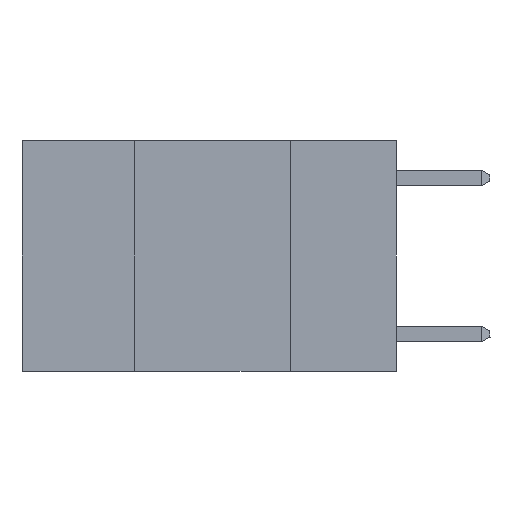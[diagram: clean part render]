
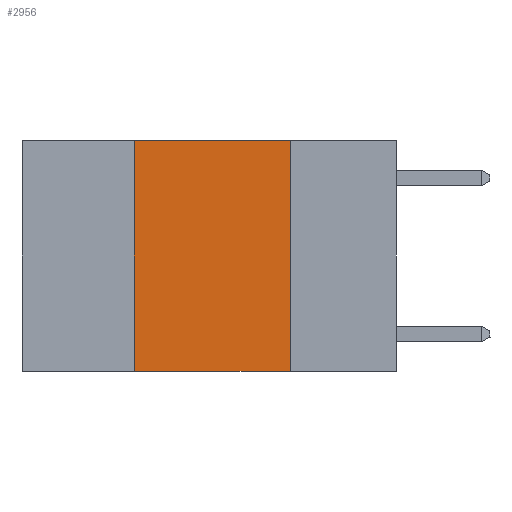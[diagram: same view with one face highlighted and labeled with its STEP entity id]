
A CAD part, left-side view. The second image highlights one B-rep face of the part: STEP entity #2956.
In plain terms, the highlighted planar face has unit normal (-1, 0, 0).
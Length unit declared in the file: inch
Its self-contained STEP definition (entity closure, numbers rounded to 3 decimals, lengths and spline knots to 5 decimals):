
#1341 = CARTESIAN_POINT ( 'NONE',  ( 0., 0.6, 0. ) ) ;
#1369 = VERTEX_POINT ( 'NONE', #6479 ) ;
#1586 = LINE ( 'NONE', #4068, #4581 ) ;
#1599 = DIRECTION ( 'NONE',  ( 0., -1., 0. ) ) ;
#1645 = ORIENTED_EDGE ( 'NONE', *, *, #8865, .F. ) ;
#2563 = EDGE_CURVE ( 'NONE', #1369, #8768, #1586, .T. ) ;
#2866 = CARTESIAN_POINT ( 'NONE',  ( 0., 0.42, 0. ) ) ;
#2956 = ADVANCED_FACE ( 'NONE', ( #5621 ), #8032, .F. ) ;
#3426 = ORIENTED_EDGE ( 'NONE', *, *, #13070, .F. ) ;
#3830 = CARTESIAN_POINT ( 'NONE',  ( 0., 0.6, 0. ) ) ;
#4057 = VECTOR ( 'NONE', #1599, 39.37008 ) ;
#4068 = CARTESIAN_POINT ( 'NONE',  ( 0., 0.6, -0.37 ) ) ;
#4373 = AXIS2_PLACEMENT_3D ( 'NONE', #1341, #11306, #4743 ) ;
#4509 = DIRECTION ( 'NONE',  ( 0., 0., -1. ) ) ;
#4581 = VECTOR ( 'NONE', #11743, 39.37008 ) ;
#4743 = DIRECTION ( 'NONE',  ( 0., 0., -1. ) ) ;
#4827 = ORIENTED_EDGE ( 'NONE', *, *, #12293, .F. ) ;
#5518 = ORIENTED_EDGE ( 'NONE', *, *, #2563, .T. ) ;
#5621 = FACE_OUTER_BOUND ( 'NONE', #9812, .T. ) ;
#6154 = CARTESIAN_POINT ( 'NONE',  ( 0., 0.42, 0. ) ) ;
#6479 = CARTESIAN_POINT ( 'NONE',  ( 0., 0.42, -0.37 ) ) ;
#7294 = DIRECTION ( 'NONE',  ( 0., 0., 1. ) ) ;
#8032 = PLANE ( 'NONE',  #4373 ) ;
#8589 = LINE ( 'NONE', #6154, #13984 ) ;
#8768 = VERTEX_POINT ( 'NONE', #10930 ) ;
#8865 = EDGE_CURVE ( 'NONE', #12990, #8768, #10222, .T. ) ;
#9812 = EDGE_LOOP ( 'NONE', ( #1645, #3426, #4827, #5518 ) ) ;
#9867 = VECTOR ( 'NONE', #4509, 39.37008 ) ;
#10222 = LINE ( 'NONE', #12190, #9867 ) ;
#10318 = CARTESIAN_POINT ( 'NONE',  ( 0., 0.17, 0. ) ) ;
#10501 = VERTEX_POINT ( 'NONE', #2866 ) ;
#10930 = CARTESIAN_POINT ( 'NONE',  ( 0., 0.17, -0.37 ) ) ;
#11306 = DIRECTION ( 'NONE',  ( 1., 0., 0. ) ) ;
#11743 = DIRECTION ( 'NONE',  ( 0., -1., 0. ) ) ;
#12190 = CARTESIAN_POINT ( 'NONE',  ( 0., 0.17, 0. ) ) ;
#12293 = EDGE_CURVE ( 'NONE', #1369, #10501, #8589, .T. ) ;
#12821 = LINE ( 'NONE', #3830, #4057 ) ;
#12990 = VERTEX_POINT ( 'NONE', #10318 ) ;
#13070 = EDGE_CURVE ( 'NONE', #10501, #12990, #12821, .T. ) ;
#13984 = VECTOR ( 'NONE', #7294, 39.37008 ) ;
